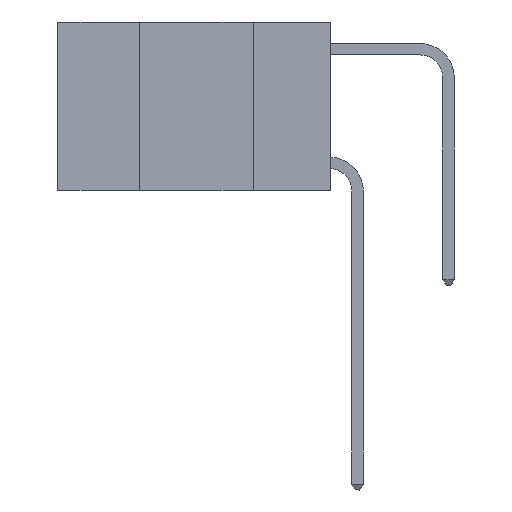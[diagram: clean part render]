
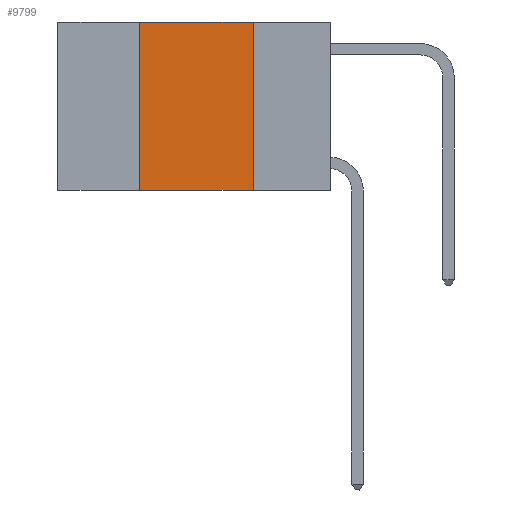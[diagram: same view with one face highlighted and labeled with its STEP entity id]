
A CAD part, left-side view. The second image highlights one B-rep face of the part: STEP entity #9799.
In plain terms, the highlighted planar face has unit normal (-1, 0, 0).
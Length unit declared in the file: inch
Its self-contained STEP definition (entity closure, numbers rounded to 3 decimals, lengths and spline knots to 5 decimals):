
#15 = LINE ( 'NONE', #13723, #2703 ) ;
#297 = VERTEX_POINT ( 'NONE', #5481 ) ;
#542 = ORIENTED_EDGE ( 'NONE', *, *, #11766, .F. ) ;
#620 = DIRECTION ( 'NONE',  ( 0., -1., 0. ) ) ;
#663 = CARTESIAN_POINT ( 'NONE',  ( 0., 0.17, 0. ) ) ;
#855 = LINE ( 'NONE', #11670, #3551 ) ;
#1066 = CARTESIAN_POINT ( 'NONE',  ( 0., 0.6, 0. ) ) ;
#2376 = VERTEX_POINT ( 'NONE', #663 ) ;
#2703 = VECTOR ( 'NONE', #12602, 39.37008 ) ;
#3366 = DIRECTION ( 'NONE',  ( 0., 0., -1. ) ) ;
#3551 = VECTOR ( 'NONE', #3716, 39.37008 ) ;
#3716 = DIRECTION ( 'NONE',  ( 0., 0., 1. ) ) ;
#4531 = CARTESIAN_POINT ( 'NONE',  ( 0., 0.42, -0.37 ) ) ;
#5481 = CARTESIAN_POINT ( 'NONE',  ( 0., 0.17, -0.37 ) ) ;
#6667 = VECTOR ( 'NONE', #620, 39.37008 ) ;
#7039 = ORIENTED_EDGE ( 'NONE', *, *, #13679, .F. ) ;
#7503 = VERTEX_POINT ( 'NONE', #4531 ) ;
#7627 = CARTESIAN_POINT ( 'NONE',  ( 0., 0.42, 0. ) ) ;
#7997 = CARTESIAN_POINT ( 'NONE',  ( 0., 0.6, -0.37 ) ) ;
#8488 = VERTEX_POINT ( 'NONE', #7627 ) ;
#9083 = PLANE ( 'NONE',  #14083 ) ;
#9085 = DIRECTION ( 'NONE',  ( 0., -1., 0. ) ) ;
#9103 = EDGE_CURVE ( 'NONE', #8488, #2376, #9663, .T. ) ;
#9663 = LINE ( 'NONE', #11971, #6667 ) ;
#9664 = ORIENTED_EDGE ( 'NONE', *, *, #9103, .F. ) ;
#9799 = ADVANCED_FACE ( 'NONE', ( #13742 ), #9083, .F. ) ;
#9863 = LINE ( 'NONE', #7997, #10207 ) ;
#10204 = DIRECTION ( 'NONE',  ( 1., 0., 0. ) ) ;
#10207 = VECTOR ( 'NONE', #9085, 39.37008 ) ;
#11057 = ORIENTED_EDGE ( 'NONE', *, *, #11687, .T. ) ;
#11670 = CARTESIAN_POINT ( 'NONE',  ( 0., 0.42, 0. ) ) ;
#11687 = EDGE_CURVE ( 'NONE', #7503, #297, #9863, .T. ) ;
#11766 = EDGE_CURVE ( 'NONE', #2376, #297, #15, .T. ) ;
#11971 = CARTESIAN_POINT ( 'NONE',  ( 0., 0.6, 0. ) ) ;
#12602 = DIRECTION ( 'NONE',  ( 0., 0., -1. ) ) ;
#13151 = EDGE_LOOP ( 'NONE', ( #542, #9664, #7039, #11057 ) ) ;
#13679 = EDGE_CURVE ( 'NONE', #7503, #8488, #855, .T. ) ;
#13723 = CARTESIAN_POINT ( 'NONE',  ( 0., 0.17, 0. ) ) ;
#13742 = FACE_OUTER_BOUND ( 'NONE', #13151, .T. ) ;
#14083 = AXIS2_PLACEMENT_3D ( 'NONE', #1066, #10204, #3366 ) ;
